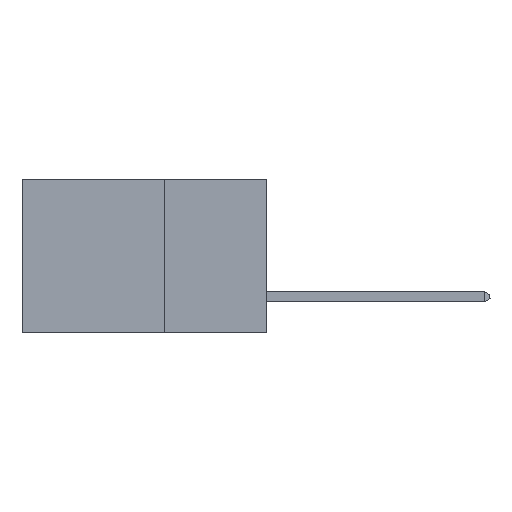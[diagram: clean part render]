
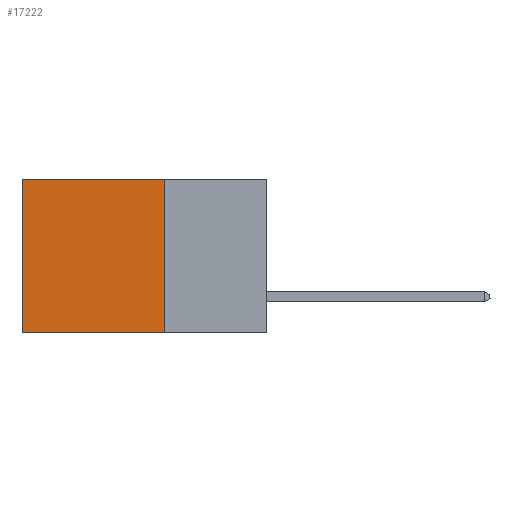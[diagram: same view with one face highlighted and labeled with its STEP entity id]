
A CAD part, left-side view. The second image highlights one B-rep face of the part: STEP entity #17222.
In plain terms, the highlighted planar face has unit normal (-1, 0, 0).
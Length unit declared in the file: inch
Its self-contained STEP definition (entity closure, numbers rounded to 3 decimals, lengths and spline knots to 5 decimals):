
#2716 = FACE_OUTER_BOUND ( 'NONE', #19672, .T. ) ;
#2990 = EDGE_CURVE ( 'NONE', #9515, #8271, #5864, .T. ) ;
#3207 = CARTESIAN_POINT ( 'NONE',  ( 0.2875, 0.6, -0.375 ) ) ;
#3381 = CARTESIAN_POINT ( 'NONE',  ( 0.2875, 0.25, -0.375 ) ) ;
#3676 = DIRECTION ( 'NONE',  ( 0., 0., -1. ) ) ;
#5864 = LINE ( 'NONE', #3207, #9164 ) ;
#6139 = CARTESIAN_POINT ( 'NONE',  ( 0.2875, 0.25, 0. ) ) ;
#6416 = VERTEX_POINT ( 'NONE', #17815 ) ;
#6966 = VECTOR ( 'NONE', #19946, 39.37008 ) ;
#6972 = LINE ( 'NONE', #19844, #13784 ) ;
#7033 = EDGE_CURVE ( 'NONE', #6416, #16131, #6972, .T. ) ;
#8124 = PLANE ( 'NONE',  #14011 ) ;
#8238 = CARTESIAN_POINT ( 'NONE',  ( 0.2875, 0.25, -0.375 ) ) ;
#8271 = VERTEX_POINT ( 'NONE', #18616 ) ;
#9164 = VECTOR ( 'NONE', #19147, 39.37008 ) ;
#9515 = VERTEX_POINT ( 'NONE', #10588 ) ;
#10101 = ORIENTED_EDGE ( 'NONE', *, *, #11582, .F. ) ;
#10588 = CARTESIAN_POINT ( 'NONE',  ( 0.2875, 0.6, 0. ) ) ;
#10734 = LINE ( 'NONE', #13294, #6966 ) ;
#11486 = DIRECTION ( 'NONE',  ( 1., 0., 0. ) ) ;
#11582 = EDGE_CURVE ( 'NONE', #16131, #8271, #10734, .T. ) ;
#11954 = ORIENTED_EDGE ( 'NONE', *, *, #17971, .T. ) ;
#13294 = CARTESIAN_POINT ( 'NONE',  ( 0.2875, 0.25, -0.375 ) ) ;
#13784 = VECTOR ( 'NONE', #3676, 39.37008 ) ;
#14001 = DIRECTION ( 'NONE',  ( 0., 1., 0. ) ) ;
#14011 = AXIS2_PLACEMENT_3D ( 'NONE', #3381, #11486, #16306 ) ;
#16131 = VERTEX_POINT ( 'NONE', #8238 ) ;
#16306 = DIRECTION ( 'NONE',  ( 0., 0., -1. ) ) ;
#17078 = ORIENTED_EDGE ( 'NONE', *, *, #7033, .F. ) ;
#17116 = VECTOR ( 'NONE', #14001, 39.37008 ) ;
#17222 = ADVANCED_FACE ( 'NONE', ( #2716 ), #8124, .F. ) ;
#17815 = CARTESIAN_POINT ( 'NONE',  ( 0.2875, 0.25, 0. ) ) ;
#17971 = EDGE_CURVE ( 'NONE', #6416, #9515, #19889, .T. ) ;
#18616 = CARTESIAN_POINT ( 'NONE',  ( 0.2875, 0.6, -0.375 ) ) ;
#19147 = DIRECTION ( 'NONE',  ( 0., 0., -1. ) ) ;
#19672 = EDGE_LOOP ( 'NONE', ( #20840, #10101, #17078, #11954 ) ) ;
#19844 = CARTESIAN_POINT ( 'NONE',  ( 0.2875, 0.25, -0.375 ) ) ;
#19889 = LINE ( 'NONE', #6139, #17116 ) ;
#19946 = DIRECTION ( 'NONE',  ( 0., 1., 0. ) ) ;
#20840 = ORIENTED_EDGE ( 'NONE', *, *, #2990, .T. ) ;
